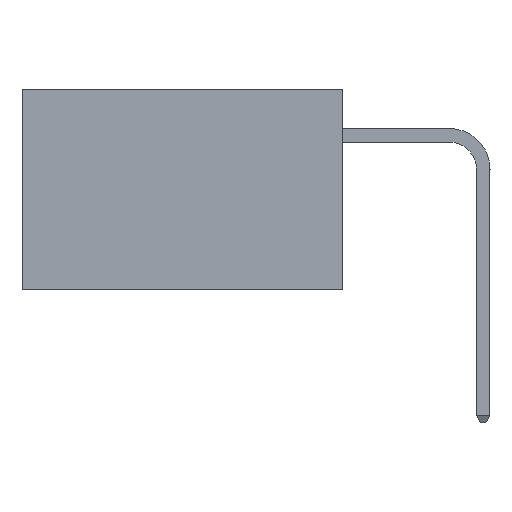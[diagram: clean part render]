
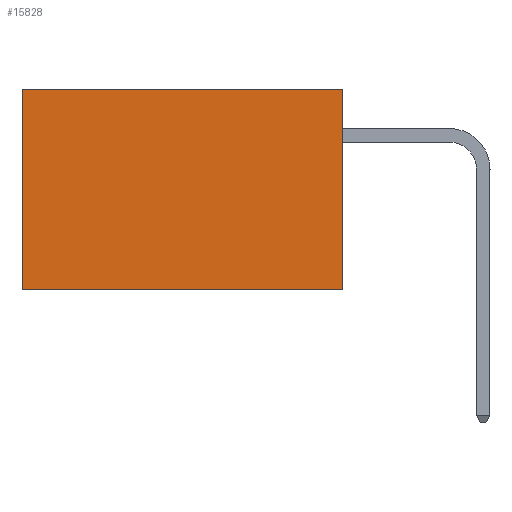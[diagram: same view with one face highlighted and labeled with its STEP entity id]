
A CAD part, left-side view. The second image highlights one B-rep face of the part: STEP entity #15828.
In plain terms, the highlighted planar face has unit normal (-1, 0, 0).
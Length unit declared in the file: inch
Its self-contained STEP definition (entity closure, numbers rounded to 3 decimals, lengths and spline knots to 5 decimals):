
#1188 = CARTESIAN_POINT ( 'NONE',  ( 0.277, 0., -0.37 ) ) ;
#1840 = EDGE_CURVE ( 'NONE', #19049, #10141, #20631, .T. ) ;
#2188 = DIRECTION ( 'NONE',  ( 0., 1., 0. ) ) ;
#2840 = VECTOR ( 'NONE', #6939, 39.37008 ) ;
#3379 = LINE ( 'NONE', #8599, #2840 ) ;
#4117 = CARTESIAN_POINT ( 'NONE',  ( 0.277, 0.59, -0.37 ) ) ;
#4255 = CARTESIAN_POINT ( 'NONE',  ( 0.277, 0.59, 0. ) ) ;
#6939 = DIRECTION ( 'NONE',  ( 0., 0., -1. ) ) ;
#7200 = ORIENTED_EDGE ( 'NONE', *, *, #14177, .F. ) ;
#7842 = VECTOR ( 'NONE', #2188, 39.37008 ) ;
#7866 = PLANE ( 'NONE',  #16348 ) ;
#8599 = CARTESIAN_POINT ( 'NONE',  ( 0.277, 0.59, -0.37 ) ) ;
#9435 = VECTOR ( 'NONE', #13842, 39.37008 ) ;
#9516 = DIRECTION ( 'NONE',  ( 0., 0., -1. ) ) ;
#9678 = CARTESIAN_POINT ( 'NONE',  ( 0.277, 0., 0. ) ) ;
#9792 = VECTOR ( 'NONE', #13306, 39.37008 ) ;
#9910 = EDGE_CURVE ( 'NONE', #10141, #19947, #3379, .T. ) ;
#10141 = VERTEX_POINT ( 'NONE', #4255 ) ;
#10794 = ORIENTED_EDGE ( 'NONE', *, *, #9910, .T. ) ;
#11241 = FACE_OUTER_BOUND ( 'NONE', #18590, .T. ) ;
#11277 = ORIENTED_EDGE ( 'NONE', *, *, #16127, .F. ) ;
#11693 = CARTESIAN_POINT ( 'NONE',  ( 0.277, 0., -0.37 ) ) ;
#13306 = DIRECTION ( 'NONE',  ( 0., 0., -1. ) ) ;
#13842 = DIRECTION ( 'NONE',  ( 0., 1., 0. ) ) ;
#14177 = EDGE_CURVE ( 'NONE', #19049, #17699, #18310, .T. ) ;
#14329 = CARTESIAN_POINT ( 'NONE',  ( 0.277, 0., -0.37 ) ) ;
#15828 = ADVANCED_FACE ( 'NONE', ( #11241 ), #7866, .F. ) ;
#15911 = ORIENTED_EDGE ( 'NONE', *, *, #1840, .T. ) ;
#16127 = EDGE_CURVE ( 'NONE', #17699, #19947, #17485, .T. ) ;
#16152 = CARTESIAN_POINT ( 'NONE',  ( 0.277, 0., 0. ) ) ;
#16348 = AXIS2_PLACEMENT_3D ( 'NONE', #1188, #19129, #9516 ) ;
#17485 = LINE ( 'NONE', #20151, #9435 ) ;
#17699 = VERTEX_POINT ( 'NONE', #14329 ) ;
#18310 = LINE ( 'NONE', #11693, #9792 ) ;
#18590 = EDGE_LOOP ( 'NONE', ( #10794, #11277, #7200, #15911 ) ) ;
#19049 = VERTEX_POINT ( 'NONE', #9678 ) ;
#19129 = DIRECTION ( 'NONE',  ( 1., 0., 0. ) ) ;
#19947 = VERTEX_POINT ( 'NONE', #4117 ) ;
#20151 = CARTESIAN_POINT ( 'NONE',  ( 0.277, 0., -0.37 ) ) ;
#20631 = LINE ( 'NONE', #16152, #7842 ) ;
